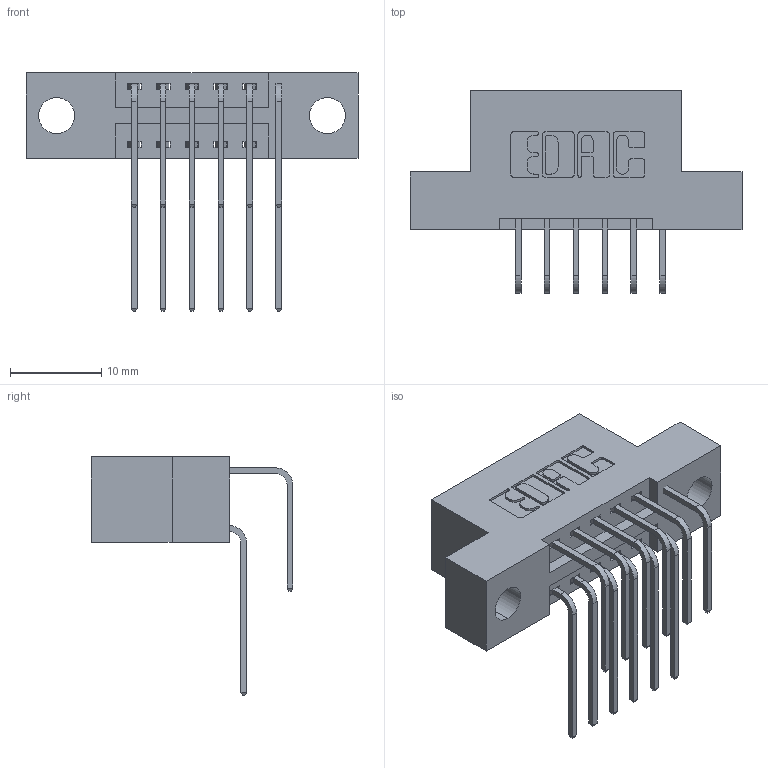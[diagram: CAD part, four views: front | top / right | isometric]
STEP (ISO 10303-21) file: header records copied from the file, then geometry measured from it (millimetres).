
FILE_DESCRIPTION (( 'STEP AP203' ), '1' );
FILE_NAME ('346-012-558-204.STEP', '2022-05-17T20:45:02', ( '' ), ( '' ), 'SwSTEP 2.0', 'SolidWorks 2020', '' );
FILE_SCHEMA (( 'CONFIG_CONTROL_DESIGN' ));
Length unit declared in the file: inch
Products named in the file (4): 346 Part_Flush Mounting Lugs - 0.156 Dia-TH; 345-292-001_558 Tail - 2; 345-292-001_558 559 Tail - 1; 346-012-558-204
Assembly tree (13 placements, depth 2):
  346-012-558-204
    346 Part_Flush Mounting Lugs - 0.156 Dia-TH
    345-292-001_558 559 Tail - 1  x6
    345-292-001_558 Tail - 2  x6
Bounding box: 36.45 x 22.16 x 26.16 mm (x, y, z)
Volume: 3248.1 mm3; surface area: 4167 mm2
Topology: 13 solids, 13 shells, 772 faces, 2255 edges, 1486 vertices
Faces by surface type: plane 524, cylinder 248
Entity records: 10511 total; most frequent: CARTESIAN_POINT 1831, ORIENTED_EDGE 1710, DIRECTION 1639, EDGE_CURVE 855, VECTOR 663, LINE 663, VERTEX_POINT 566, AXIS2_PLACEMENT_3D 488
